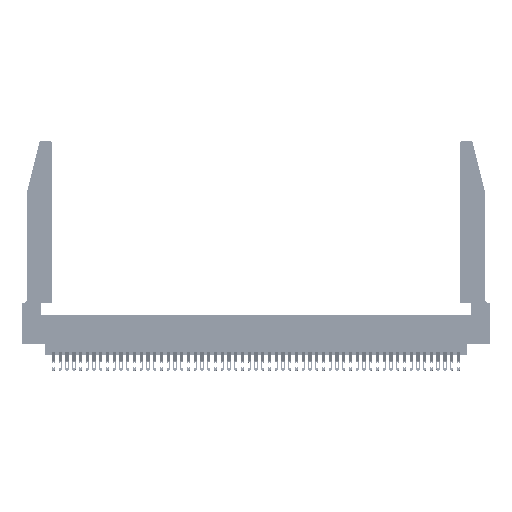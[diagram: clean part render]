
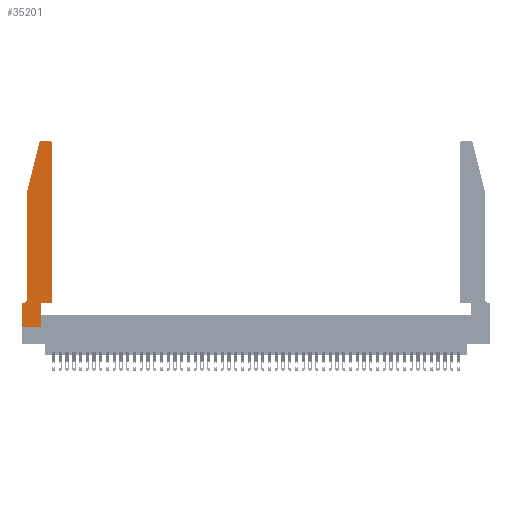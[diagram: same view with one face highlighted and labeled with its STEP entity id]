
A CAD part, top view. The second image highlights one B-rep face of the part: STEP entity #35201.
In plain terms, the highlighted planar face has unit normal (0, 0, 1).
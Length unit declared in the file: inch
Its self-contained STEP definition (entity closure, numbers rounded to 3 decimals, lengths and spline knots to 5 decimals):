
#363 = CIRCLE ( 'NONE', #33443, 0.03 ) ;
#588 = CARTESIAN_POINT ( 'NONE',  ( 0.0055, 0.42, 0.37 ) ) ;
#633 = LINE ( 'NONE', #21548, #47055 ) ;
#1841 = VERTEX_POINT ( 'NONE', #3629 ) ;
#2019 = CARTESIAN_POINT ( 'NONE',  ( 0.25487, 2.72718, 0.37 ) ) ;
#2244 = VECTOR ( 'NONE', #7711, 39.37008 ) ;
#3229 = VECTOR ( 'NONE', #3292, 39.37008 ) ;
#3292 = DIRECTION ( 'NONE',  ( 1., 0., 0. ) ) ;
#3614 = VERTEX_POINT ( 'NONE', #16085 ) ;
#3629 = CARTESIAN_POINT ( 'NONE',  ( 0.0055, 0.35, 0.37 ) ) ;
#6275 = VECTOR ( 'NONE', #49496, 39.37008 ) ;
#6418 = EDGE_CURVE ( 'NONE', #47117, #40494, #14848, .T. ) ;
#6448 = VERTEX_POINT ( 'NONE', #2019 ) ;
#6714 = EDGE_CURVE ( 'NONE', #14772, #46101, #13585, .T. ) ;
#7199 = VECTOR ( 'NONE', #28162, 39.37008 ) ;
#7711 = DIRECTION ( 'NONE',  ( 0., -1., 0. ) ) ;
#8070 = VERTEX_POINT ( 'NONE', #9957 ) ;
#8299 = DIRECTION ( 'NONE',  ( 0., 0., -1. ) ) ;
#8388 = LINE ( 'NONE', #27128, #2244 ) ;
#9435 = CARTESIAN_POINT ( 'NONE',  ( 0.4505, 2.72, 0.37 ) ) ;
#9859 = CARTESIAN_POINT ( 'NONE',  ( 0.0755, 0.35, 0.37 ) ) ;
#9895 = DIRECTION ( 'NONE',  ( 1., 0., 0. ) ) ;
#9921 = LINE ( 'NONE', #23722, #50173 ) ;
#9957 = CARTESIAN_POINT ( 'NONE',  ( 0.284, 2.75, 0.37 ) ) ;
#10031 = VERTEX_POINT ( 'NONE', #35303 ) ;
#10063 = DIRECTION ( 'NONE',  ( 0., 0., 1. ) ) ;
#10236 = PLANE ( 'NONE',  #48885 ) ;
#10924 = ORIENTED_EDGE ( 'NONE', *, *, #23131, .T. ) ;
#11277 = EDGE_CURVE ( 'NONE', #33952, #1841, #40627, .T. ) ;
#11718 = CARTESIAN_POINT ( 'NONE',  ( 0.2865, 0., 0.37 ) ) ;
#13026 = ORIENTED_EDGE ( 'NONE', *, *, #20080, .T. ) ;
#13252 = CARTESIAN_POINT ( 'NONE',  ( 0.4505, 0.35, 0.37 ) ) ;
#13276 = AXIS2_PLACEMENT_3D ( 'NONE', #48926, #10063, #17707 ) ;
#13562 = VERTEX_POINT ( 'NONE', #50377 ) ;
#13585 = LINE ( 'NONE', #13252, #40408 ) ;
#13623 = CARTESIAN_POINT ( 'NONE',  ( 0.4205, 2.72, 0.37 ) ) ;
#13969 = DIRECTION ( 'NONE',  ( 0., 0., 1. ) ) ;
#14772 = VERTEX_POINT ( 'NONE', #23300 ) ;
#14848 = LINE ( 'NONE', #19453, #27026 ) ;
#15587 = EDGE_CURVE ( 'NONE', #40494, #14772, #28231, .T. ) ;
#16085 = CARTESIAN_POINT ( 'NONE',  ( 0.0755, 2., 0.37 ) ) ;
#16578 = ORIENTED_EDGE ( 'NONE', *, *, #6714, .T. ) ;
#16634 = LINE ( 'NONE', #29333, #6275 ) ;
#17475 = CIRCLE ( 'NONE', #13276, 0.03 ) ;
#17707 = DIRECTION ( 'NONE',  ( 1., 0., 0. ) ) ;
#17821 = ORIENTED_EDGE ( 'NONE', *, *, #18371, .T. ) ;
#18371 = EDGE_CURVE ( 'NONE', #1841, #38122, #32209, .T. ) ;
#18891 = EDGE_CURVE ( 'NONE', #3614, #33952, #16634, .T. ) ;
#19445 = AXIS2_PLACEMENT_3D ( 'NONE', #588, #8299, #47523 ) ;
#19453 = CARTESIAN_POINT ( 'NONE',  ( 0.2865, 0.35, 0.37 ) ) ;
#19625 = ORIENTED_EDGE ( 'NONE', *, *, #6418, .T. ) ;
#20080 = EDGE_CURVE ( 'NONE', #6448, #3614, #633, .T. ) ;
#20255 = ORIENTED_EDGE ( 'NONE', *, *, #34793, .T. ) ;
#20636 = VECTOR ( 'NONE', #25670, 39.37008 ) ;
#20956 = DIRECTION ( 'NONE',  ( 0., 1., 0. ) ) ;
#21203 = LINE ( 'NONE', #40940, #7199 ) ;
#21548 = CARTESIAN_POINT ( 'NONE',  ( 0.0755, 2., 0.37 ) ) ;
#21783 = DIRECTION ( 'NONE',  ( 0., 0., 1. ) ) ;
#21948 = CARTESIAN_POINT ( 'NONE',  ( 0., 0.35, 0.37 ) ) ;
#23131 = EDGE_CURVE ( 'NONE', #8070, #6448, #17475, .T. ) ;
#23300 = CARTESIAN_POINT ( 'NONE',  ( 0.4505, 0.35, 0.37 ) ) ;
#23722 = CARTESIAN_POINT ( 'NONE',  ( 0., 0., 0.37 ) ) ;
#25298 = CARTESIAN_POINT ( 'NONE',  ( 0.0755, 0.42, 0.37 ) ) ;
#25546 = DIRECTION ( 'NONE',  ( 1., 0., 0. ) ) ;
#25670 = DIRECTION ( 'NONE',  ( -1., 0., 0. ) ) ;
#27026 = VECTOR ( 'NONE', #20956, 39.37008 ) ;
#27128 = CARTESIAN_POINT ( 'NONE',  ( 0., 0., 0.37 ) ) ;
#28162 = DIRECTION ( 'NONE',  ( -1., 0., 0. ) ) ;
#28231 = LINE ( 'NONE', #34614, #3229 ) ;
#29333 = CARTESIAN_POINT ( 'NONE',  ( 0.0755, 2., 0.37 ) ) ;
#30394 = CARTESIAN_POINT ( 'NONE',  ( 0.2865, 0.35, 0.37 ) ) ;
#32209 = LINE ( 'NONE', #9859, #20636 ) ;
#32261 = ORIENTED_EDGE ( 'NONE', *, *, #15587, .T. ) ;
#33443 = AXIS2_PLACEMENT_3D ( 'NONE', #13623, #21783, #25546 ) ;
#33952 = VERTEX_POINT ( 'NONE', #25298 ) ;
#34388 = EDGE_LOOP ( 'NONE', ( #42492, #10924, #13026, #35062, #41752, #17821, #20255, #47254, #19625, #32261, #16578, #46407 ) ) ;
#34488 = EDGE_CURVE ( 'NONE', #10031, #8070, #21203, .T. ) ;
#34614 = CARTESIAN_POINT ( 'NONE',  ( 0.4505, 0.35, 0.37 ) ) ;
#34793 = EDGE_CURVE ( 'NONE', #38122, #13562, #8388, .T. ) ;
#35062 = ORIENTED_EDGE ( 'NONE', *, *, #18891, .T. ) ;
#35147 = EDGE_CURVE ( 'NONE', #46101, #10031, #363, .T. ) ;
#35201 = ADVANCED_FACE ( 'NONE', ( #48588 ), #10236, .T. ) ;
#35303 = CARTESIAN_POINT ( 'NONE',  ( 0.4205, 2.75, 0.37 ) ) ;
#36495 = DIRECTION ( 'NONE',  ( 1., 0., 0. ) ) ;
#38122 = VERTEX_POINT ( 'NONE', #43222 ) ;
#40408 = VECTOR ( 'NONE', #40487, 39.37008 ) ;
#40487 = DIRECTION ( 'NONE',  ( 0., 1., 0. ) ) ;
#40494 = VERTEX_POINT ( 'NONE', #30394 ) ;
#40627 = CIRCLE ( 'NONE', #19445, 0.07 ) ;
#40940 = CARTESIAN_POINT ( 'NONE',  ( 0.2605, 2.75, 0.37 ) ) ;
#41752 = ORIENTED_EDGE ( 'NONE', *, *, #11277, .T. ) ;
#42492 = ORIENTED_EDGE ( 'NONE', *, *, #34488, .T. ) ;
#43222 = CARTESIAN_POINT ( 'NONE',  ( 0., 0.35, 0.37 ) ) ;
#44774 = DIRECTION ( 'NONE',  ( -0.239, -0.971, 0. ) ) ;
#46101 = VERTEX_POINT ( 'NONE', #9435 ) ;
#46407 = ORIENTED_EDGE ( 'NONE', *, *, #35147, .T. ) ;
#47055 = VECTOR ( 'NONE', #44774, 39.37008 ) ;
#47117 = VERTEX_POINT ( 'NONE', #11718 ) ;
#47254 = ORIENTED_EDGE ( 'NONE', *, *, #48024, .T. ) ;
#47523 = DIRECTION ( 'NONE',  ( -1., 0., 0. ) ) ;
#48024 = EDGE_CURVE ( 'NONE', #13562, #47117, #9921, .T. ) ;
#48588 = FACE_OUTER_BOUND ( 'NONE', #34388, .T. ) ;
#48885 = AXIS2_PLACEMENT_3D ( 'NONE', #21948, #13969, #9895 ) ;
#48926 = CARTESIAN_POINT ( 'NONE',  ( 0.284, 2.72, 0.37 ) ) ;
#49496 = DIRECTION ( 'NONE',  ( 0., -1., 0. ) ) ;
#50173 = VECTOR ( 'NONE', #36495, 39.37008 ) ;
#50377 = CARTESIAN_POINT ( 'NONE',  ( 0., 0., 0.37 ) ) ;
